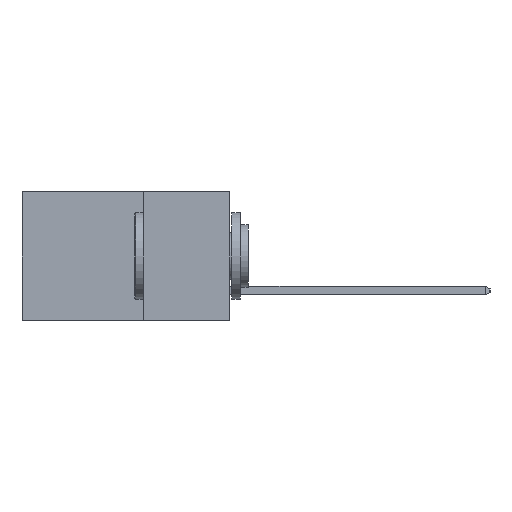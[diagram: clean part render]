
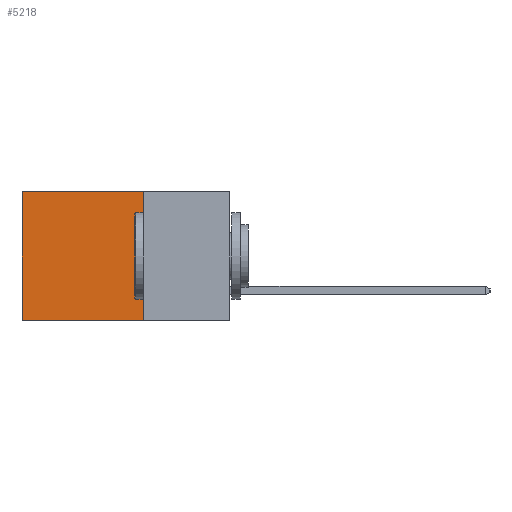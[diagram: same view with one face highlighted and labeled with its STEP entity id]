
A CAD part, left-side view. The second image highlights one B-rep face of the part: STEP entity #5218.
In plain terms, the highlighted planar face has unit normal (-1, 0, 0).
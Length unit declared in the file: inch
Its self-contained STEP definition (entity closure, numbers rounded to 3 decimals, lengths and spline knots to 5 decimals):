
#668 = EDGE_CURVE ( 'NONE', #15775, #15057, #12663, .T. ) ;
#893 = LINE ( 'NONE', #15971, #21838 ) ;
#2046 = AXIS2_PLACEMENT_3D ( 'NONE', #4349, #4246, #4217 ) ;
#4217 = DIRECTION ( 'NONE',  ( 0., 0., -1. ) ) ;
#4246 = DIRECTION ( 'NONE',  ( 1., 0., 0. ) ) ;
#4349 = CARTESIAN_POINT ( 'NONE',  ( 0.2615, 0.25, -0.37 ) ) ;
#4421 = PLANE ( 'NONE',  #2046 ) ;
#4888 = CARTESIAN_POINT ( 'NONE',  ( 0.2615, 0.25, -0.37 ) ) ;
#5218 = ADVANCED_FACE ( 'NONE', ( #8069 ), #4421, .F. ) ;
#5593 = CARTESIAN_POINT ( 'NONE',  ( 0.2615, 0.6, -0.37 ) ) ;
#8069 = FACE_OUTER_BOUND ( 'NONE', #22333, .T. ) ;
#8304 = ORIENTED_EDGE ( 'NONE', *, *, #13304, .F. ) ;
#8514 = EDGE_CURVE ( 'NONE', #15775, #20999, #25773, .T. ) ;
#9344 = DIRECTION ( 'NONE',  ( 0., 1., 0. ) ) ;
#10187 = ORIENTED_EDGE ( 'NONE', *, *, #18522, .T. ) ;
#12663 = LINE ( 'NONE', #18367, #18753 ) ;
#13304 = EDGE_CURVE ( 'NONE', #15057, #13576, #893, .T. ) ;
#13576 = VERTEX_POINT ( 'NONE', #22769 ) ;
#14444 = ORIENTED_EDGE ( 'NONE', *, *, #8514, .T. ) ;
#15057 = VERTEX_POINT ( 'NONE', #4888 ) ;
#15224 = CARTESIAN_POINT ( 'NONE',  ( 0.2615, 0.25, 0. ) ) ;
#15356 = CARTESIAN_POINT ( 'NONE',  ( 0.2615, 0.25, 0. ) ) ;
#15775 = VERTEX_POINT ( 'NONE', #15224 ) ;
#15788 = DIRECTION ( 'NONE',  ( 0., 0., -1. ) ) ;
#15971 = CARTESIAN_POINT ( 'NONE',  ( 0.2615, 0.25, -0.37 ) ) ;
#16061 = DIRECTION ( 'NONE',  ( 0., 1., 0. ) ) ;
#16267 = VECTOR ( 'NONE', #15788, 39.37008 ) ;
#16908 = LINE ( 'NONE', #5593, #16267 ) ;
#17969 = DIRECTION ( 'NONE',  ( 0., 0., -1. ) ) ;
#18367 = CARTESIAN_POINT ( 'NONE',  ( 0.2615, 0.25, -0.37 ) ) ;
#18522 = EDGE_CURVE ( 'NONE', #20999, #13576, #16908, .T. ) ;
#18753 = VECTOR ( 'NONE', #17969, 39.37008 ) ;
#20573 = VECTOR ( 'NONE', #9344, 39.37008 ) ;
#20962 = ORIENTED_EDGE ( 'NONE', *, *, #668, .F. ) ;
#20999 = VERTEX_POINT ( 'NONE', #24611 ) ;
#21838 = VECTOR ( 'NONE', #16061, 39.37008 ) ;
#22333 = EDGE_LOOP ( 'NONE', ( #10187, #8304, #20962, #14444 ) ) ;
#22769 = CARTESIAN_POINT ( 'NONE',  ( 0.2615, 0.6, -0.37 ) ) ;
#24611 = CARTESIAN_POINT ( 'NONE',  ( 0.2615, 0.6, 0. ) ) ;
#25773 = LINE ( 'NONE', #15356, #20573 ) ;
